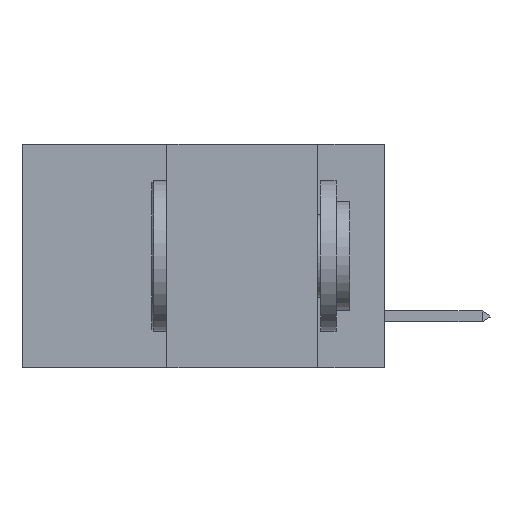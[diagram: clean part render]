
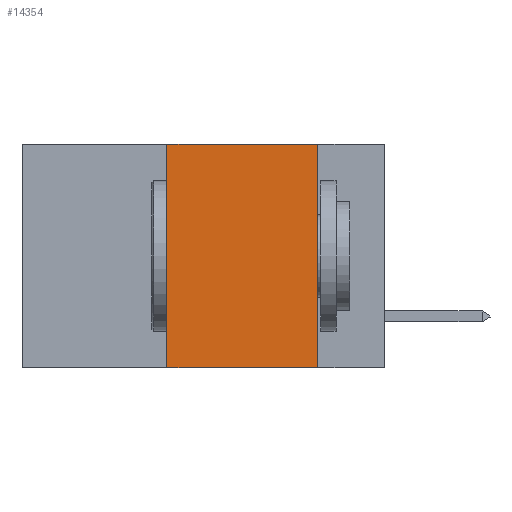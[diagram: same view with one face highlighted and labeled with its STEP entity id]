
A CAD part, left-side view. The second image highlights one B-rep face of the part: STEP entity #14354.
In plain terms, the highlighted planar face has unit normal (-1, 0, 0).
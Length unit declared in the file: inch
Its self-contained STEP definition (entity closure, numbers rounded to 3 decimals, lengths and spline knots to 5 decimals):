
#933 = CARTESIAN_POINT ( 'NONE',  ( 0., 0.36, 0. ) ) ;
#1452 = DIRECTION ( 'NONE',  ( 0., 0., -1. ) ) ;
#4499 = CARTESIAN_POINT ( 'NONE',  ( 0., 0.11, -0.37 ) ) ;
#6336 = PLANE ( 'NONE',  #16284 ) ;
#7153 = VERTEX_POINT ( 'NONE', #15843 ) ;
#7314 = ORIENTED_EDGE ( 'NONE', *, *, #8616, .F. ) ;
#8616 = EDGE_CURVE ( 'NONE', #19198, #13082, #13806, .T. ) ;
#9509 = EDGE_CURVE ( 'NONE', #13082, #30291, #13919, .T. ) ;
#9628 = DIRECTION ( 'NONE',  ( 0., 0., -1. ) ) ;
#13082 = VERTEX_POINT ( 'NONE', #25789 ) ;
#13240 = FACE_OUTER_BOUND ( 'NONE', #23206, .T. ) ;
#13806 = LINE ( 'NONE', #35983, #21338 ) ;
#13919 = LINE ( 'NONE', #20644, #28501 ) ;
#14354 = ADVANCED_FACE ( 'NONE', ( #13240 ), #6336, .F. ) ;
#15843 = CARTESIAN_POINT ( 'NONE',  ( 0., 0.36, -0.37 ) ) ;
#16284 = AXIS2_PLACEMENT_3D ( 'NONE', #41561, #28844, #9628 ) ;
#18746 = LINE ( 'NONE', #23267, #28766 ) ;
#19198 = VERTEX_POINT ( 'NONE', #26634 ) ;
#20644 = CARTESIAN_POINT ( 'NONE',  ( 0., 0.11, 0. ) ) ;
#20833 = DIRECTION ( 'NONE',  ( 0., 0., 1. ) ) ;
#20907 = EDGE_CURVE ( 'NONE', #7153, #30291, #18746, .T. ) ;
#21338 = VECTOR ( 'NONE', #29356, 39.37008 ) ;
#23206 = EDGE_LOOP ( 'NONE', ( #39946, #7314, #41775, #29121 ) ) ;
#23267 = CARTESIAN_POINT ( 'NONE',  ( 0., 0.6, -0.37 ) ) ;
#23537 = VECTOR ( 'NONE', #20833, 39.37008 ) ;
#25789 = CARTESIAN_POINT ( 'NONE',  ( 0., 0.11, 0. ) ) ;
#26275 = EDGE_CURVE ( 'NONE', #7153, #19198, #40669, .T. ) ;
#26634 = CARTESIAN_POINT ( 'NONE',  ( 0., 0.36, 0. ) ) ;
#28501 = VECTOR ( 'NONE', #1452, 39.37008 ) ;
#28766 = VECTOR ( 'NONE', #32415, 39.37008 ) ;
#28844 = DIRECTION ( 'NONE',  ( 1., 0., 0. ) ) ;
#29121 = ORIENTED_EDGE ( 'NONE', *, *, #20907, .T. ) ;
#29356 = DIRECTION ( 'NONE',  ( 0., -1., 0. ) ) ;
#30291 = VERTEX_POINT ( 'NONE', #4499 ) ;
#32415 = DIRECTION ( 'NONE',  ( 0., -1., 0. ) ) ;
#35983 = CARTESIAN_POINT ( 'NONE',  ( 0., 0.6, 0. ) ) ;
#39946 = ORIENTED_EDGE ( 'NONE', *, *, #9509, .F. ) ;
#40669 = LINE ( 'NONE', #933, #23537 ) ;
#41561 = CARTESIAN_POINT ( 'NONE',  ( 0., 0.6, 0. ) ) ;
#41775 = ORIENTED_EDGE ( 'NONE', *, *, #26275, .F. ) ;
